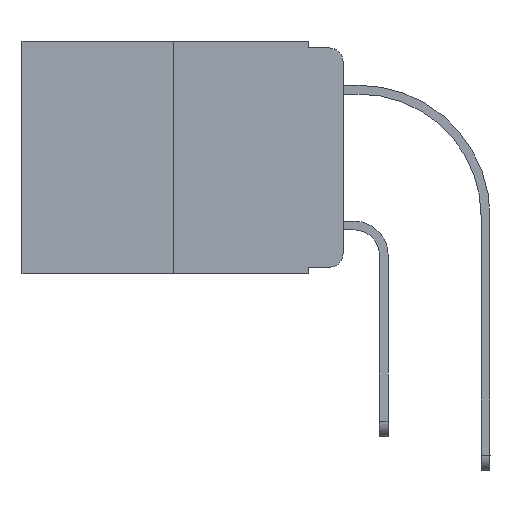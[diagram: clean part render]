
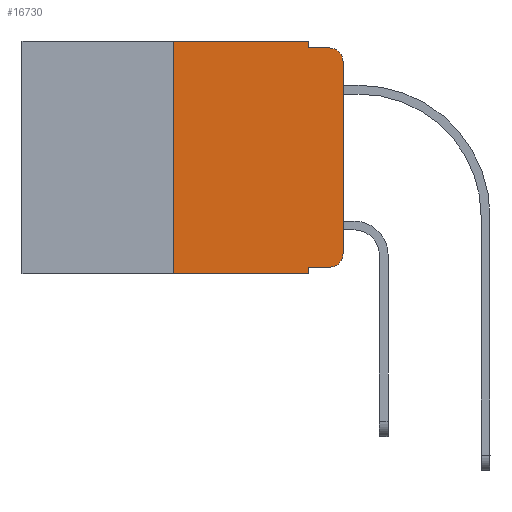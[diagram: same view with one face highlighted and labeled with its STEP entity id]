
A CAD part, left-side view. The second image highlights one B-rep face of the part: STEP entity #16730.
In plain terms, the highlighted planar face has unit normal (-1, 0, 0).
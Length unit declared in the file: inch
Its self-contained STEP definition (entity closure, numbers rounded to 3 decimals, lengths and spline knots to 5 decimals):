
#267 = CARTESIAN_POINT ( 'NONE',  ( 0., 0.051, -0.343 ) ) ;
#665 = AXIS2_PLACEMENT_3D ( 'NONE', #6705, #18373, #5280 ) ;
#873 = CARTESIAN_POINT ( 'NONE',  ( 0., 0.25, -0.343 ) ) ;
#918 = DIRECTION ( 'NONE',  ( 0., 0., -1. ) ) ;
#1438 = CARTESIAN_POINT ( 'NONE',  ( 0., 0.25, 0. ) ) ;
#1831 = ORIENTED_EDGE ( 'NONE', *, *, #18057, .T. ) ;
#1844 = EDGE_CURVE ( 'NONE', #4751, #12562, #8828, .T. ) ;
#1869 = FACE_OUTER_BOUND ( 'NONE', #9941, .T. ) ;
#2627 = CARTESIAN_POINT ( 'NONE',  ( 0., 0.051, -0.01 ) ) ;
#2750 = CARTESIAN_POINT ( 'NONE',  ( 0., 0.051, 0. ) ) ;
#2920 = CARTESIAN_POINT ( 'NONE',  ( 0., 0.473, -0.343 ) ) ;
#3145 = VECTOR ( 'NONE', #15317, 39.37008 ) ;
#3159 = EDGE_CURVE ( 'NONE', #4751, #8163, #7109, .T. ) ;
#3208 = DIRECTION ( 'NONE',  ( 0., 0., 1. ) ) ;
#3262 = ORIENTED_EDGE ( 'NONE', *, *, #4315, .T. ) ;
#3574 = VERTEX_POINT ( 'NONE', #10235 ) ;
#3604 = VECTOR ( 'NONE', #3208, 39.37008 ) ;
#3684 = VERTEX_POINT ( 'NONE', #14552 ) ;
#4138 = CARTESIAN_POINT ( 'NONE',  ( 0., 0.051, 0. ) ) ;
#4315 = EDGE_CURVE ( 'NONE', #3684, #3574, #5966, .T. ) ;
#4608 = LINE ( 'NONE', #10158, #9309 ) ;
#4751 = VERTEX_POINT ( 'NONE', #873 ) ;
#4938 = CARTESIAN_POINT ( 'NONE',  ( 0., 0., -0.03 ) ) ;
#5153 = ORIENTED_EDGE ( 'NONE', *, *, #3159, .T. ) ;
#5216 = CARTESIAN_POINT ( 'NONE',  ( 0., 0.051, 0. ) ) ;
#5280 = DIRECTION ( 'NONE',  ( 0., 0., -1. ) ) ;
#5342 = VERTEX_POINT ( 'NONE', #2627 ) ;
#5424 = CARTESIAN_POINT ( 'NONE',  ( 0., 0.051, -0.333 ) ) ;
#5966 = CIRCLE ( 'NONE', #9929, 0.02 ) ;
#6168 = CARTESIAN_POINT ( 'NONE',  ( 0., 0.25, 0. ) ) ;
#6705 = CARTESIAN_POINT ( 'NONE',  ( 0., 0.02, -0.03 ) ) ;
#7031 = DIRECTION ( 'NONE',  ( 0., -1., 0. ) ) ;
#7109 = LINE ( 'NONE', #2920, #17577 ) ;
#7887 = LINE ( 'NONE', #5424, #17560 ) ;
#7954 = LINE ( 'NONE', #18006, #3145 ) ;
#8091 = LINE ( 'NONE', #17168, #14731 ) ;
#8163 = VERTEX_POINT ( 'NONE', #267 ) ;
#8558 = DIRECTION ( 'NONE',  ( 0., 0., -1. ) ) ;
#8628 = DIRECTION ( 'NONE',  ( 0., -1., 0. ) ) ;
#8828 = LINE ( 'NONE', #6168, #3604 ) ;
#8894 = CIRCLE ( 'NONE', #665, 0.02 ) ;
#9223 = DIRECTION ( 'NONE',  ( 1., 0., 0. ) ) ;
#9309 = VECTOR ( 'NONE', #18870, 39.37008 ) ;
#9589 = ORIENTED_EDGE ( 'NONE', *, *, #10047, .T. ) ;
#9929 = AXIS2_PLACEMENT_3D ( 'NONE', #18443, #13929, #918 ) ;
#9941 = EDGE_LOOP ( 'NONE', ( #9589, #1831, #10169, #12693, #14398, #10405, #5153, #11973, #16103, #3262 ) ) ;
#9956 = DIRECTION ( 'NONE',  ( 0., 0., -1. ) ) ;
#10047 = EDGE_CURVE ( 'NONE', #3574, #16916, #8091, .T. ) ;
#10158 = CARTESIAN_POINT ( 'NONE',  ( 0., 0.473, 0. ) ) ;
#10169 = ORIENTED_EDGE ( 'NONE', *, *, #17453, .F. ) ;
#10235 = CARTESIAN_POINT ( 'NONE',  ( 0., 0., -0.313 ) ) ;
#10405 = ORIENTED_EDGE ( 'NONE', *, *, #1844, .F. ) ;
#10803 = VECTOR ( 'NONE', #9956, 39.37008 ) ;
#10922 = VERTEX_POINT ( 'NONE', #13872 ) ;
#11189 = EDGE_CURVE ( 'NONE', #10922, #8163, #11447, .T. ) ;
#11447 = LINE ( 'NONE', #2750, #15355 ) ;
#11584 = VERTEX_POINT ( 'NONE', #5216 ) ;
#11973 = ORIENTED_EDGE ( 'NONE', *, *, #11189, .F. ) ;
#12256 = AXIS2_PLACEMENT_3D ( 'NONE', #16498, #9223, #13348 ) ;
#12562 = VERTEX_POINT ( 'NONE', #1438 ) ;
#12693 = ORIENTED_EDGE ( 'NONE', *, *, #13666, .F. ) ;
#12786 = EDGE_CURVE ( 'NONE', #10922, #3684, #7887, .T. ) ;
#13335 = VERTEX_POINT ( 'NONE', #17701 ) ;
#13348 = DIRECTION ( 'NONE',  ( 0., 0., -1. ) ) ;
#13666 = EDGE_CURVE ( 'NONE', #11584, #5342, #16951, .T. ) ;
#13872 = CARTESIAN_POINT ( 'NONE',  ( 0., 0.051, -0.333 ) ) ;
#13929 = DIRECTION ( 'NONE',  ( -1., 0., 0. ) ) ;
#14298 = DIRECTION ( 'NONE',  ( 0., 0., 1. ) ) ;
#14398 = ORIENTED_EDGE ( 'NONE', *, *, #14560, .F. ) ;
#14552 = CARTESIAN_POINT ( 'NONE',  ( 0., 0.02, -0.333 ) ) ;
#14560 = EDGE_CURVE ( 'NONE', #12562, #11584, #4608, .T. ) ;
#14686 = PLANE ( 'NONE',  #12256 ) ;
#14731 = VECTOR ( 'NONE', #14298, 39.37008 ) ;
#15317 = DIRECTION ( 'NONE',  ( 0., -1., 0. ) ) ;
#15355 = VECTOR ( 'NONE', #8558, 39.37008 ) ;
#16103 = ORIENTED_EDGE ( 'NONE', *, *, #12786, .T. ) ;
#16498 = CARTESIAN_POINT ( 'NONE',  ( 0., 0.473, 0. ) ) ;
#16730 = ADVANCED_FACE ( 'NONE', ( #1869 ), #14686, .F. ) ;
#16916 = VERTEX_POINT ( 'NONE', #4938 ) ;
#16951 = LINE ( 'NONE', #4138, #10803 ) ;
#17168 = CARTESIAN_POINT ( 'NONE',  ( 0., 0., 0. ) ) ;
#17453 = EDGE_CURVE ( 'NONE', #5342, #13335, #7954, .T. ) ;
#17560 = VECTOR ( 'NONE', #7031, 39.37008 ) ;
#17577 = VECTOR ( 'NONE', #8628, 39.37008 ) ;
#17701 = CARTESIAN_POINT ( 'NONE',  ( 0., 0.02, -0.01 ) ) ;
#18006 = CARTESIAN_POINT ( 'NONE',  ( 0., 0.051, -0.01 ) ) ;
#18057 = EDGE_CURVE ( 'NONE', #16916, #13335, #8894, .T. ) ;
#18373 = DIRECTION ( 'NONE',  ( -1., 0., 0. ) ) ;
#18443 = CARTESIAN_POINT ( 'NONE',  ( 0., 0.02, -0.313 ) ) ;
#18870 = DIRECTION ( 'NONE',  ( 0., -1., 0. ) ) ;
